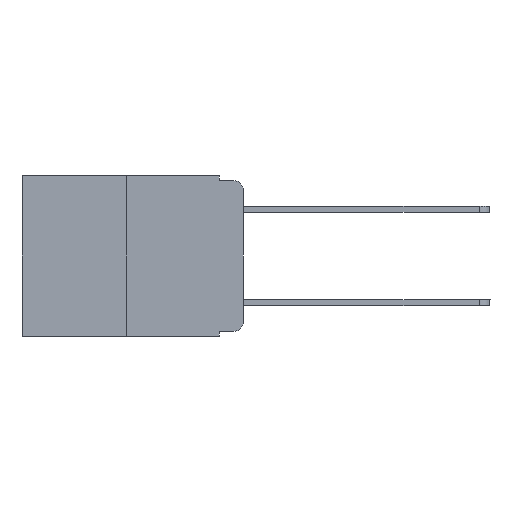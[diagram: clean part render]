
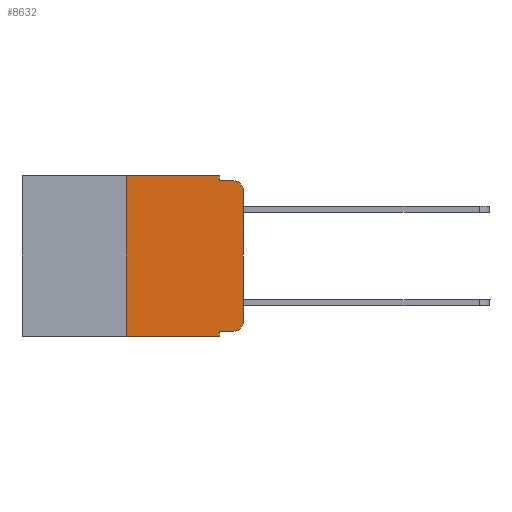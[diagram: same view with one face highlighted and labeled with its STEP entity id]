
A CAD part, left-side view. The second image highlights one B-rep face of the part: STEP entity #8632.
In plain terms, the highlighted planar face has unit normal (-1, 0, 0).
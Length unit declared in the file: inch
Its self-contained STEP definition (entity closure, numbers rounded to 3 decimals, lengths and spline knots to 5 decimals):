
#202 = CIRCLE ( 'NONE', #5509, 0.02 ) ;
#689 = DIRECTION ( 'NONE',  ( 0., 0., -1. ) ) ;
#956 = LINE ( 'NONE', #10641, #11917 ) ;
#1216 = FACE_OUTER_BOUND ( 'NONE', #11039, .T. ) ;
#1231 = VERTEX_POINT ( 'NONE', #7659 ) ;
#1617 = VERTEX_POINT ( 'NONE', #3872 ) ;
#1749 = VERTEX_POINT ( 'NONE', #2949 ) ;
#1991 = LINE ( 'NONE', #2039, #12961 ) ;
#2039 = CARTESIAN_POINT ( 'NONE',  ( 0., 0.473, -0.343 ) ) ;
#2076 = VERTEX_POINT ( 'NONE', #8381 ) ;
#2154 = VERTEX_POINT ( 'NONE', #11496 ) ;
#2254 = EDGE_CURVE ( 'NONE', #1617, #2154, #956, .T. ) ;
#2458 = AXIS2_PLACEMENT_3D ( 'NONE', #9360, #11587, #11413 ) ;
#2478 = ORIENTED_EDGE ( 'NONE', *, *, #10787, .T. ) ;
#2602 = VECTOR ( 'NONE', #7770, 39.37008 ) ;
#2731 = EDGE_CURVE ( 'NONE', #2076, #5769, #10264, .T. ) ;
#2781 = ORIENTED_EDGE ( 'NONE', *, *, #2254, .F. ) ;
#2900 = VECTOR ( 'NONE', #3036, 39.37008 ) ;
#2949 = CARTESIAN_POINT ( 'NONE',  ( 0., 0.02, -0.333 ) ) ;
#2995 = LINE ( 'NONE', #10730, #3958 ) ;
#3036 = DIRECTION ( 'NONE',  ( 0., -1., 0. ) ) ;
#3207 = CARTESIAN_POINT ( 'NONE',  ( 0., 0.25, -0.343 ) ) ;
#3290 = DIRECTION ( 'NONE',  ( 0., 0., -1. ) ) ;
#3325 = CARTESIAN_POINT ( 'NONE',  ( 0., 0.051, -0.333 ) ) ;
#3374 = DIRECTION ( 'NONE',  ( 0., -1., 0. ) ) ;
#3476 = ORIENTED_EDGE ( 'NONE', *, *, #11566, .T. ) ;
#3623 = ORIENTED_EDGE ( 'NONE', *, *, #5373, .F. ) ;
#3651 = VERTEX_POINT ( 'NONE', #6502 ) ;
#3872 = CARTESIAN_POINT ( 'NONE',  ( 0., 0.25, 0. ) ) ;
#3887 = VECTOR ( 'NONE', #6464, 39.37008 ) ;
#3958 = VECTOR ( 'NONE', #3290, 39.37008 ) ;
#4165 = DIRECTION ( 'NONE',  ( 0., 0., -1. ) ) ;
#4728 = ORIENTED_EDGE ( 'NONE', *, *, #12273, .T. ) ;
#5219 = CARTESIAN_POINT ( 'NONE',  ( 0., 0.051, -0.333 ) ) ;
#5373 = EDGE_CURVE ( 'NONE', #2154, #2076, #9085, .T. ) ;
#5383 = CARTESIAN_POINT ( 'NONE',  ( 0., 0.051, -0.343 ) ) ;
#5509 = AXIS2_PLACEMENT_3D ( 'NONE', #6015, #12541, #9493 ) ;
#5562 = DIRECTION ( 'NONE',  ( 0., 0., 1. ) ) ;
#5769 = VERTEX_POINT ( 'NONE', #9884 ) ;
#6015 = CARTESIAN_POINT ( 'NONE',  ( 0., 0.02, -0.313 ) ) ;
#6274 = PLANE ( 'NONE',  #11242 ) ;
#6341 = LINE ( 'NONE', #9811, #2602 ) ;
#6464 = DIRECTION ( 'NONE',  ( 0., -1., 0. ) ) ;
#6502 = CARTESIAN_POINT ( 'NONE',  ( 0., 0., -0.03 ) ) ;
#6505 = VERTEX_POINT ( 'NONE', #5219 ) ;
#6524 = CARTESIAN_POINT ( 'NONE',  ( 0., 0.473, 0. ) ) ;
#6819 = EDGE_CURVE ( 'NONE', #3651, #5769, #7374, .T. ) ;
#7199 = LINE ( 'NONE', #3325, #3887 ) ;
#7210 = VERTEX_POINT ( 'NONE', #5383 ) ;
#7366 = ORIENTED_EDGE ( 'NONE', *, *, #9665, .F. ) ;
#7374 = CIRCLE ( 'NONE', #2458, 0.02 ) ;
#7519 = LINE ( 'NONE', #7677, #10175 ) ;
#7659 = CARTESIAN_POINT ( 'NONE',  ( 0., 0., -0.313 ) ) ;
#7677 = CARTESIAN_POINT ( 'NONE',  ( 0., 0.25, 0. ) ) ;
#7770 = DIRECTION ( 'NONE',  ( 0., 0., 1. ) ) ;
#8076 = VECTOR ( 'NONE', #4165, 39.37008 ) ;
#8381 = CARTESIAN_POINT ( 'NONE',  ( 0., 0.051, -0.01 ) ) ;
#8632 = ADVANCED_FACE ( 'NONE', ( #1216 ), #6274, .F. ) ;
#9085 = LINE ( 'NONE', #13566, #8076 ) ;
#9289 = VERTEX_POINT ( 'NONE', #3207 ) ;
#9360 = CARTESIAN_POINT ( 'NONE',  ( 0., 0.02, -0.03 ) ) ;
#9493 = DIRECTION ( 'NONE',  ( 0., 0., -1. ) ) ;
#9514 = EDGE_CURVE ( 'NONE', #1749, #1231, #202, .T. ) ;
#9665 = EDGE_CURVE ( 'NONE', #6505, #7210, #2995, .T. ) ;
#9811 = CARTESIAN_POINT ( 'NONE',  ( 0., 0., 0. ) ) ;
#9884 = CARTESIAN_POINT ( 'NONE',  ( 0., 0.02, -0.01 ) ) ;
#10175 = VECTOR ( 'NONE', #5562, 39.37008 ) ;
#10261 = ORIENTED_EDGE ( 'NONE', *, *, #10995, .F. ) ;
#10264 = LINE ( 'NONE', #11431, #2900 ) ;
#10641 = CARTESIAN_POINT ( 'NONE',  ( 0., 0.473, 0. ) ) ;
#10730 = CARTESIAN_POINT ( 'NONE',  ( 0., 0.051, 0. ) ) ;
#10787 = EDGE_CURVE ( 'NONE', #9289, #7210, #1991, .T. ) ;
#10995 = EDGE_CURVE ( 'NONE', #9289, #1617, #7519, .T. ) ;
#11039 = EDGE_LOOP ( 'NONE', ( #4728, #12956, #11503, #3623, #2781, #10261, #2478, #7366, #3476, #12396 ) ) ;
#11242 = AXIS2_PLACEMENT_3D ( 'NONE', #6524, #12653, #689 ) ;
#11334 = DIRECTION ( 'NONE',  ( 0., -1., 0. ) ) ;
#11413 = DIRECTION ( 'NONE',  ( 0., 0., -1. ) ) ;
#11431 = CARTESIAN_POINT ( 'NONE',  ( 0., 0.051, -0.01 ) ) ;
#11496 = CARTESIAN_POINT ( 'NONE',  ( 0., 0.051, 0. ) ) ;
#11503 = ORIENTED_EDGE ( 'NONE', *, *, #2731, .F. ) ;
#11566 = EDGE_CURVE ( 'NONE', #6505, #1749, #7199, .T. ) ;
#11587 = DIRECTION ( 'NONE',  ( -1., 0., 0. ) ) ;
#11917 = VECTOR ( 'NONE', #3374, 39.37008 ) ;
#12273 = EDGE_CURVE ( 'NONE', #1231, #3651, #6341, .T. ) ;
#12396 = ORIENTED_EDGE ( 'NONE', *, *, #9514, .T. ) ;
#12541 = DIRECTION ( 'NONE',  ( -1., 0., 0. ) ) ;
#12653 = DIRECTION ( 'NONE',  ( 1., 0., 0. ) ) ;
#12956 = ORIENTED_EDGE ( 'NONE', *, *, #6819, .T. ) ;
#12961 = VECTOR ( 'NONE', #11334, 39.37008 ) ;
#13566 = CARTESIAN_POINT ( 'NONE',  ( 0., 0.051, 0. ) ) ;
